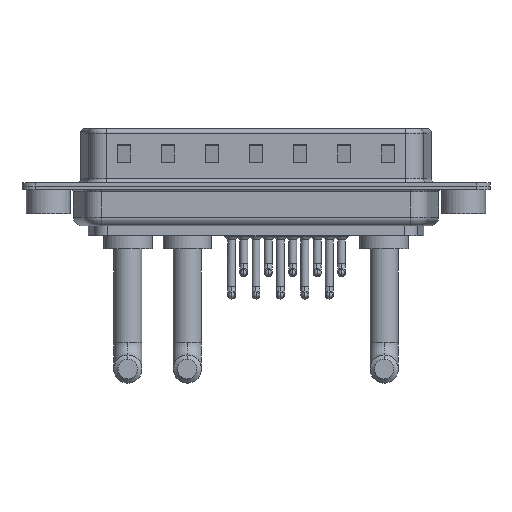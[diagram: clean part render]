
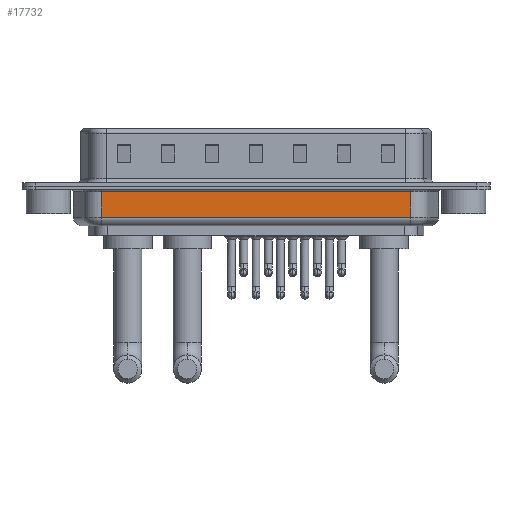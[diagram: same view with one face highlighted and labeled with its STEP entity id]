
A CAD part, front view. The second image highlights one B-rep face of the part: STEP entity #17732.
In plain terms, the highlighted planar face has unit normal (0, -1, 0).
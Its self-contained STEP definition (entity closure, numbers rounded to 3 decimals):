
#595 = DIRECTION ( 'NONE',  ( 0., 1., 0. ) ) ;
#878 = CARTESIAN_POINT ( 'NONE',  ( 6.006, -5.35, -4.5 ) ) ;
#2230 = CARTESIAN_POINT ( 'NONE',  ( 6.006, -5.35, -0.65 ) ) ;
#3715 = CARTESIAN_POINT ( 'NONE',  ( 41.044, -5.35, -3.5 ) ) ;
#3976 = VERTEX_POINT ( 'NONE', #3715 ) ;
#4420 = FACE_OUTER_BOUND ( 'NONE', #17486, .T. ) ;
#5446 = DIRECTION ( 'NONE',  ( 1., 0., 0. ) ) ;
#6181 = DIRECTION ( 'NONE',  ( -1., 0., 0. ) ) ;
#6653 = CARTESIAN_POINT ( 'NONE',  ( 6.006, -5.35, -3.5 ) ) ;
#8185 = DIRECTION ( 'NONE',  ( 0., 0., 1. ) ) ;
#9121 = VERTEX_POINT ( 'NONE', #12460 ) ;
#9275 = ORIENTED_EDGE ( 'NONE', *, *, #18223, .T. ) ;
#9557 = DIRECTION ( 'NONE',  ( 0., 0., 1. ) ) ;
#10539 = ORIENTED_EDGE ( 'NONE', *, *, #11554, .T. ) ;
#10934 = AXIS2_PLACEMENT_3D ( 'NONE', #18761, #595, #9557 ) ;
#11435 = LINE ( 'NONE', #2230, #14781 ) ;
#11554 = EDGE_CURVE ( 'NONE', #3976, #9121, #21320, .T. ) ;
#11588 = PLANE ( 'NONE',  #10934 ) ;
#11873 = LINE ( 'NONE', #878, #17563 ) ;
#12460 = CARTESIAN_POINT ( 'NONE',  ( 41.044, -5.35, -0.65 ) ) ;
#14779 = VECTOR ( 'NONE', #5446, 1000. ) ;
#14781 = VECTOR ( 'NONE', #6181, 1000. ) ;
#15000 = ORIENTED_EDGE ( 'NONE', *, *, #19672, .T. ) ;
#16323 = LINE ( 'NONE', #20027, #14779 ) ;
#17248 = DIRECTION ( 'NONE',  ( 0., 0., 1. ) ) ;
#17486 = EDGE_LOOP ( 'NONE', ( #18119, #15000, #10539, #9275 ) ) ;
#17563 = VECTOR ( 'NONE', #17248, 1000. ) ;
#17732 = ADVANCED_FACE ( 'NONE', ( #4420 ), #11588, .F. ) ;
#18119 = ORIENTED_EDGE ( 'NONE', *, *, #22377, .F. ) ;
#18223 = EDGE_CURVE ( 'NONE', #9121, #21530, #11435, .T. ) ;
#18761 = CARTESIAN_POINT ( 'NONE',  ( 6.006, -5.35, -4.5 ) ) ;
#19443 = VERTEX_POINT ( 'NONE', #6653 ) ;
#19672 = EDGE_CURVE ( 'NONE', #19443, #3976, #16323, .T. ) ;
#20027 = CARTESIAN_POINT ( 'NONE',  ( 6.006, -5.35, -3.5 ) ) ;
#20353 = VECTOR ( 'NONE', #8185, 1000. ) ;
#21320 = LINE ( 'NONE', #22883, #20353 ) ;
#21530 = VERTEX_POINT ( 'NONE', #22840 ) ;
#22377 = EDGE_CURVE ( 'NONE', #19443, #21530, #11873, .T. ) ;
#22840 = CARTESIAN_POINT ( 'NONE',  ( 6.006, -5.35, -0.65 ) ) ;
#22883 = CARTESIAN_POINT ( 'NONE',  ( 41.044, -5.35, -4.5 ) ) ;
